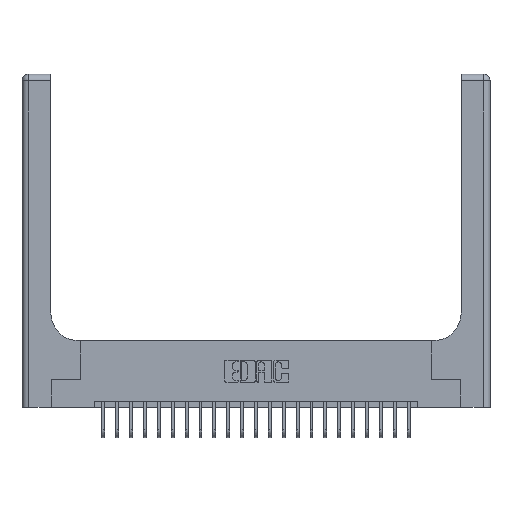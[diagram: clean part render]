
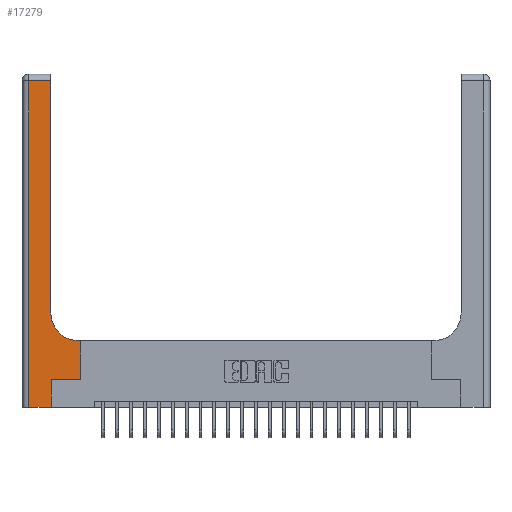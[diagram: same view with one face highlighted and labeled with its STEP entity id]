
A CAD part, top view. The second image highlights one B-rep face of the part: STEP entity #17279.
In plain terms, the highlighted planar face has unit normal (0, 0, 1).
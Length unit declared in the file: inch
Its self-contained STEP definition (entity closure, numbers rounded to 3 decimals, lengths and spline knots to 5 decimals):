
#637 = EDGE_CURVE ( 'NONE', #11277, #1910, #18441, .T. ) ;
#661 = CARTESIAN_POINT ( 'NONE',  ( 0.265, 0., 0.37 ) ) ;
#854 = DIRECTION ( 'NONE',  ( 0., -1., 0. ) ) ;
#1347 = CARTESIAN_POINT ( 'NONE',  ( 0.265, 0.25, 0.37 ) ) ;
#1764 = EDGE_CURVE ( 'NONE', #21711, #20675, #12856, .T. ) ;
#1910 = VERTEX_POINT ( 'NONE', #1959 ) ;
#1959 = CARTESIAN_POINT ( 'NONE',  ( 0.51, 0.6, 0.37 ) ) ;
#2166 = VERTEX_POINT ( 'NONE', #4402 ) ;
#2698 = VECTOR ( 'NONE', #4335, 39.37008 ) ;
#3313 = LINE ( 'NONE', #18407, #6799 ) ;
#3339 = DIRECTION ( 'NONE',  ( -1., 0., 0. ) ) ;
#3617 = AXIS2_PLACEMENT_3D ( 'NONE', #22077, #13595, #3339 ) ;
#3725 = VECTOR ( 'NONE', #854, 39.37008 ) ;
#3891 = EDGE_CURVE ( 'NONE', #11605, #11277, #5773, .T. ) ;
#4335 = DIRECTION ( 'NONE',  ( -1., 0., 0. ) ) ;
#4402 = CARTESIAN_POINT ( 'NONE',  ( 0.265, 0., 0.37 ) ) ;
#4621 = EDGE_CURVE ( 'NONE', #2166, #8415, #16933, .T. ) ;
#4628 = DIRECTION ( 'NONE',  ( 0., 1., 0. ) ) ;
#4708 = CIRCLE ( 'NONE', #4862, 0.25 ) ;
#4813 = VECTOR ( 'NONE', #20020, 39.37008 ) ;
#4862 = AXIS2_PLACEMENT_3D ( 'NONE', #9659, #21576, #11400 ) ;
#5077 = CARTESIAN_POINT ( 'NONE',  ( 0.528, 0.6, 0.37 ) ) ;
#5349 = EDGE_CURVE ( 'NONE', #20675, #2166, #12146, .T. ) ;
#5567 = CARTESIAN_POINT ( 'NONE',  ( 0.06, 0., 0.37 ) ) ;
#5773 = LINE ( 'NONE', #13166, #9809 ) ;
#5963 = CARTESIAN_POINT ( 'NONE',  ( 0.26, 0.85, 0.37 ) ) ;
#6799 = VECTOR ( 'NONE', #9944, 39.37008 ) ;
#8415 = VERTEX_POINT ( 'NONE', #1347 ) ;
#8754 = ORIENTED_EDGE ( 'NONE', *, *, #18490, .T. ) ;
#9132 = ORIENTED_EDGE ( 'NONE', *, *, #5349, .T. ) ;
#9659 = CARTESIAN_POINT ( 'NONE',  ( 0.51, 0.85, 0.37 ) ) ;
#9696 = DIRECTION ( 'NONE',  ( 1., 0., 0. ) ) ;
#9809 = VECTOR ( 'NONE', #4628, 39.37008 ) ;
#9944 = DIRECTION ( 'NONE',  ( 0., 1., 0. ) ) ;
#9988 = LINE ( 'NONE', #21604, #13969 ) ;
#10422 = EDGE_CURVE ( 'NONE', #8415, #11605, #9988, .T. ) ;
#10953 = EDGE_CURVE ( 'NONE', #15888, #21711, #11828, .T. ) ;
#11010 = CARTESIAN_POINT ( 'NONE',  ( 0.528, 0.25, 0.37 ) ) ;
#11277 = VERTEX_POINT ( 'NONE', #5077 ) ;
#11400 = DIRECTION ( 'NONE',  ( 1., 0., 0. ) ) ;
#11605 = VERTEX_POINT ( 'NONE', #11010 ) ;
#11828 = LINE ( 'NONE', #14568, #2698 ) ;
#12146 = LINE ( 'NONE', #19747, #20662 ) ;
#12649 = DIRECTION ( 'NONE',  ( 0., 1., 0. ) ) ;
#12856 = LINE ( 'NONE', #21408, #3725 ) ;
#13166 = CARTESIAN_POINT ( 'NONE',  ( 0.528, 0.25, 0.37 ) ) ;
#13595 = DIRECTION ( 'NONE',  ( 0., 0., -1. ) ) ;
#13641 = EDGE_CURVE ( 'NONE', #1910, #14221, #4708, .T. ) ;
#13969 = VECTOR ( 'NONE', #9696, 39.37008 ) ;
#14221 = VERTEX_POINT ( 'NONE', #5963 ) ;
#14568 = CARTESIAN_POINT ( 'NONE',  ( 0., 2.94, 0.37 ) ) ;
#15706 = ORIENTED_EDGE ( 'NONE', *, *, #10953, .T. ) ;
#15866 = ORIENTED_EDGE ( 'NONE', *, *, #1764, .T. ) ;
#15888 = VERTEX_POINT ( 'NONE', #16377 ) ;
#16377 = CARTESIAN_POINT ( 'NONE',  ( 0.26, 2.94, 0.37 ) ) ;
#16912 = PLANE ( 'NONE',  #3617 ) ;
#16933 = LINE ( 'NONE', #661, #21507 ) ;
#17279 = ADVANCED_FACE ( 'NONE', ( #18813 ), #16912, .F. ) ;
#17771 = EDGE_LOOP ( 'NONE', ( #8754, #15706, #15866, #9132, #19560, #22100, #19859, #21549, #19450 ) ) ;
#18407 = CARTESIAN_POINT ( 'NONE',  ( 0.26, 3., 0.37 ) ) ;
#18441 = LINE ( 'NONE', #21737, #4813 ) ;
#18490 = EDGE_CURVE ( 'NONE', #14221, #15888, #3313, .T. ) ;
#18585 = CARTESIAN_POINT ( 'NONE',  ( 0.06, 2.94, 0.37 ) ) ;
#18813 = FACE_OUTER_BOUND ( 'NONE', #17771, .T. ) ;
#19450 = ORIENTED_EDGE ( 'NONE', *, *, #13641, .T. ) ;
#19560 = ORIENTED_EDGE ( 'NONE', *, *, #4621, .T. ) ;
#19747 = CARTESIAN_POINT ( 'NONE',  ( 0., 0., 0.37 ) ) ;
#19859 = ORIENTED_EDGE ( 'NONE', *, *, #3891, .T. ) ;
#20020 = DIRECTION ( 'NONE',  ( -1., 0., 0. ) ) ;
#20662 = VECTOR ( 'NONE', #21476, 39.37008 ) ;
#20675 = VERTEX_POINT ( 'NONE', #5567 ) ;
#21408 = CARTESIAN_POINT ( 'NONE',  ( 0.06, 3., 0.37 ) ) ;
#21476 = DIRECTION ( 'NONE',  ( 1., 0., 0. ) ) ;
#21507 = VECTOR ( 'NONE', #12649, 39.37008 ) ;
#21549 = ORIENTED_EDGE ( 'NONE', *, *, #637, .T. ) ;
#21576 = DIRECTION ( 'NONE',  ( 0., 0., -1. ) ) ;
#21604 = CARTESIAN_POINT ( 'NONE',  ( 0.265, 0.25, 0.37 ) ) ;
#21711 = VERTEX_POINT ( 'NONE', #18585 ) ;
#21737 = CARTESIAN_POINT ( 'NONE',  ( 0.26, 0.6, 0.37 ) ) ;
#22077 = CARTESIAN_POINT ( 'NONE',  ( 0., 3., 0.37 ) ) ;
#22100 = ORIENTED_EDGE ( 'NONE', *, *, #10422, .T. ) ;
